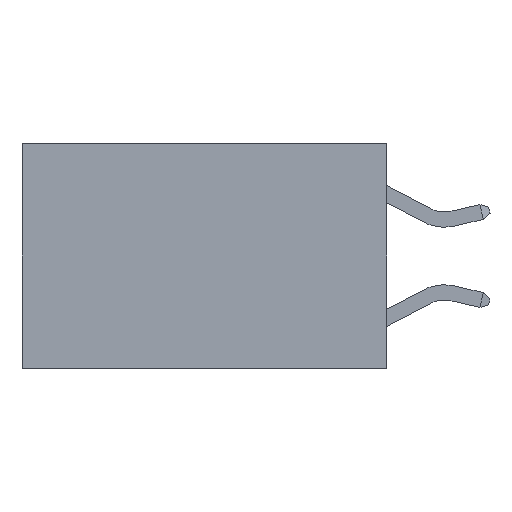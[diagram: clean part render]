
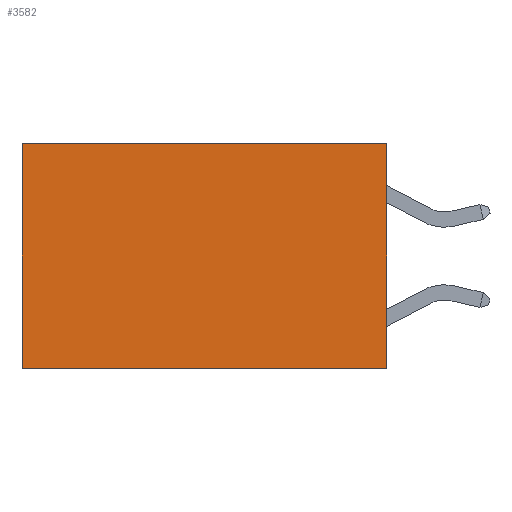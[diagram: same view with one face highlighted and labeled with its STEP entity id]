
A CAD part, left-side view. The second image highlights one B-rep face of the part: STEP entity #3582.
In plain terms, the highlighted planar face has unit normal (-1, 0, 0).
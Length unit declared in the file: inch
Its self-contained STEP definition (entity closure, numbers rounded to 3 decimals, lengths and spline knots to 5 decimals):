
#1138 = EDGE_CURVE ( 'NONE', #28098, #6409, #19785, .T. ) ;
#3022 = VECTOR ( 'NONE', #24210, 39.37008 ) ;
#3582 = ADVANCED_FACE ( 'NONE', ( #20194 ), #5999, .F. ) ;
#4022 = AXIS2_PLACEMENT_3D ( 'NONE', #12866, #24455, #13332 ) ;
#4130 = ORIENTED_EDGE ( 'NONE', *, *, #6334, .T. ) ;
#4436 = LINE ( 'NONE', #11972, #6575 ) ;
#5127 = ORIENTED_EDGE ( 'NONE', *, *, #21055, .F. ) ;
#5202 = DIRECTION ( 'NONE',  ( 0., 1., 0. ) ) ;
#5739 = VERTEX_POINT ( 'NONE', #11530 ) ;
#5782 = CARTESIAN_POINT ( 'NONE',  ( 0.2625, 0.6, 0. ) ) ;
#5999 = PLANE ( 'NONE',  #4022 ) ;
#6334 = EDGE_CURVE ( 'NONE', #6409, #5739, #17281, .T. ) ;
#6409 = VERTEX_POINT ( 'NONE', #5782 ) ;
#6575 = VECTOR ( 'NONE', #5202, 39.37008 ) ;
#7486 = VERTEX_POINT ( 'NONE', #15135 ) ;
#8263 = DIRECTION ( 'NONE',  ( 0., 0., -1. ) ) ;
#9923 = CARTESIAN_POINT ( 'NONE',  ( 0.2625, 0.6, 0. ) ) ;
#10103 = EDGE_CURVE ( 'NONE', #28098, #7486, #20182, .T. ) ;
#11530 = CARTESIAN_POINT ( 'NONE',  ( 0.2625, 0.6, -0.37 ) ) ;
#11630 = CARTESIAN_POINT ( 'NONE',  ( 0.2625, 0., 0. ) ) ;
#11972 = CARTESIAN_POINT ( 'NONE',  ( 0.2625, 0., -0.37 ) ) ;
#12866 = CARTESIAN_POINT ( 'NONE',  ( 0.2625, 0., 0. ) ) ;
#13332 = DIRECTION ( 'NONE',  ( 0., 0., -1. ) ) ;
#14449 = VECTOR ( 'NONE', #8263, 39.37008 ) ;
#15135 = CARTESIAN_POINT ( 'NONE',  ( 0.2625, 0., -0.37 ) ) ;
#16612 = DIRECTION ( 'NONE',  ( 0., 1., 0. ) ) ;
#17281 = LINE ( 'NONE', #9923, #14449 ) ;
#19476 = CARTESIAN_POINT ( 'NONE',  ( 0.2625, 0., 0. ) ) ;
#19785 = LINE ( 'NONE', #22829, #26711 ) ;
#20182 = LINE ( 'NONE', #19476, #3022 ) ;
#20194 = FACE_OUTER_BOUND ( 'NONE', #28020, .T. ) ;
#20413 = ORIENTED_EDGE ( 'NONE', *, *, #10103, .F. ) ;
#21055 = EDGE_CURVE ( 'NONE', #7486, #5739, #4436, .T. ) ;
#22829 = CARTESIAN_POINT ( 'NONE',  ( 0.2625, 0., 0. ) ) ;
#24210 = DIRECTION ( 'NONE',  ( 0., 0., -1. ) ) ;
#24455 = DIRECTION ( 'NONE',  ( 1., 0., 0. ) ) ;
#25470 = ORIENTED_EDGE ( 'NONE', *, *, #1138, .T. ) ;
#26711 = VECTOR ( 'NONE', #16612, 39.37008 ) ;
#28020 = EDGE_LOOP ( 'NONE', ( #4130, #5127, #20413, #25470 ) ) ;
#28098 = VERTEX_POINT ( 'NONE', #11630 ) ;
